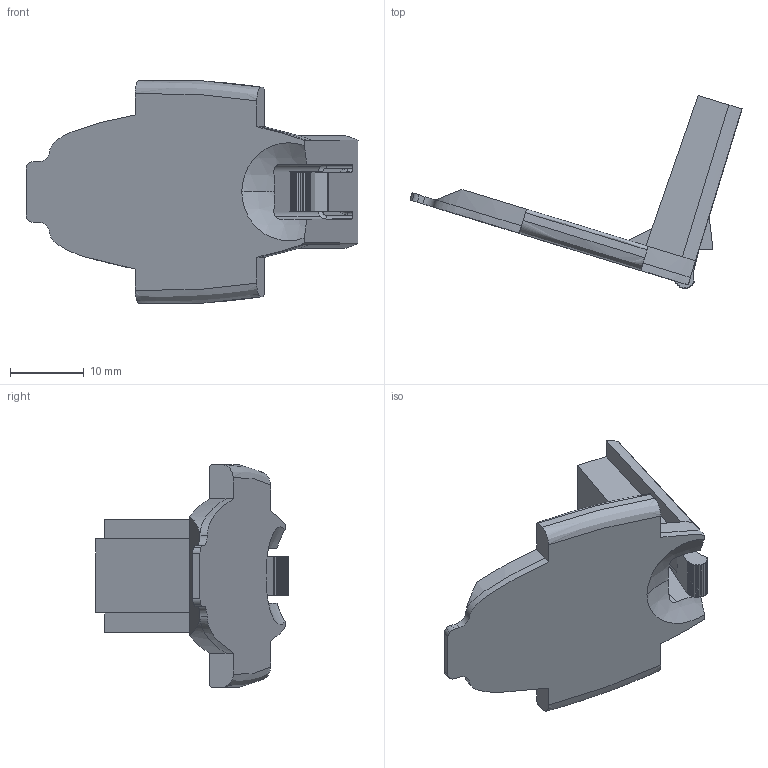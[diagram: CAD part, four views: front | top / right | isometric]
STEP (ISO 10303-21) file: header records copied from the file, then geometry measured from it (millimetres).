
FILE_DESCRIPTION (( 'STEP AP203' ), '1' );
FILE_NAME ('MOE_baseplate.STEP', '2022-01-21T14:03:49', ( '' ), ( '' ), 'SwSTEP 2.0', 'SolidWorks 2021', '' );
FILE_SCHEMA (( 'CONFIG_CONTROL_DESIGN' ));
Length unit declared in the file: inch
Products named in the file (1): MOE_baseplate
Bounding box: 44.91 x 26.08 x 30.23 mm (x, y, z)
Volume: 3823.3 mm3; surface area: 3495 mm2
Topology: 1 solids, 1 shells, 131 faces, 388 edges, 259 vertices
Faces by surface type: cylinder 61, plane 45, bspline 21, sphere 2, torus 2
Entity records: 5710 total; most frequent: CARTESIAN_POINT 2267, ORIENTED_EDGE 776, DIRECTION 632, EDGE_CURVE 388, VERTEX_POINT 259, AXIS2_PLACEMENT_3D 233, LINE 166, VECTOR 166
